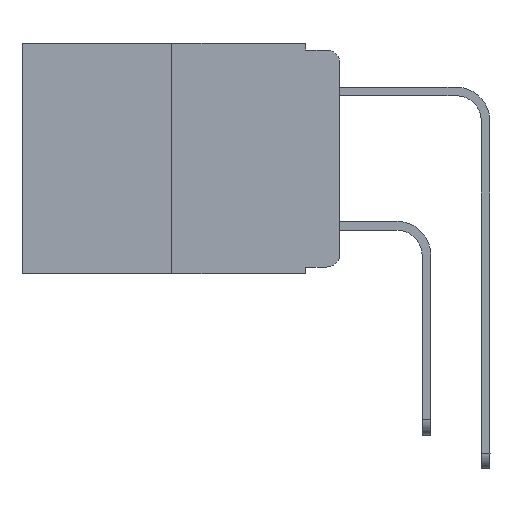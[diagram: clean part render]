
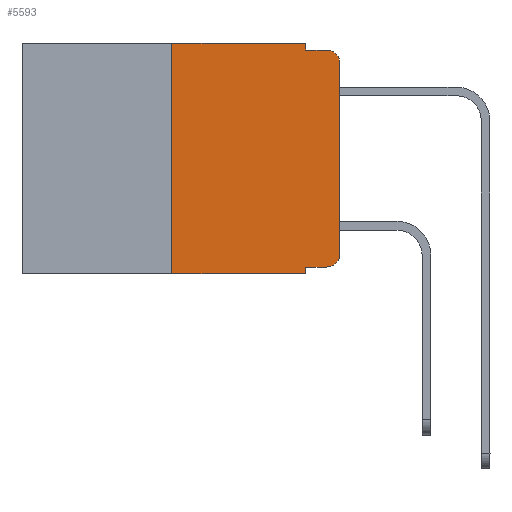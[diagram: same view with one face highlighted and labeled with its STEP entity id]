
A CAD part, left-side view. The second image highlights one B-rep face of the part: STEP entity #5593.
In plain terms, the highlighted planar face has unit normal (-1, 0, 0).
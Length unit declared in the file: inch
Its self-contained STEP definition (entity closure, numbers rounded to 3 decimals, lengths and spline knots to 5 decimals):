
#84 = PLANE ( 'NONE',  #6915 ) ;
#262 = CARTESIAN_POINT ( 'NONE',  ( 0., 0.473, 0. ) ) ;
#278 = DIRECTION ( 'NONE',  ( 0., 0., -1. ) ) ;
#373 = DIRECTION ( 'NONE',  ( 0., 0., 1. ) ) ;
#785 = CARTESIAN_POINT ( 'NONE',  ( 0., 0.473, 0. ) ) ;
#858 = CARTESIAN_POINT ( 'NONE',  ( 0., 0.051, -0.333 ) ) ;
#1084 = CARTESIAN_POINT ( 'NONE',  ( 0., 0., -0.313 ) ) ;
#1629 = LINE ( 'NONE', #12684, #1762 ) ;
#1762 = VECTOR ( 'NONE', #373, 39.37008 ) ;
#1849 = DIRECTION ( 'NONE',  ( 0., 0., -1. ) ) ;
#1924 = VERTEX_POINT ( 'NONE', #5169 ) ;
#2230 = EDGE_CURVE ( 'NONE', #6513, #14766, #7653, .T. ) ;
#2248 = VECTOR ( 'NONE', #9145, 39.37008 ) ;
#2743 = EDGE_CURVE ( 'NONE', #1924, #9829, #5109, .T. ) ;
#2850 = VERTEX_POINT ( 'NONE', #15155 ) ;
#2897 = ORIENTED_EDGE ( 'NONE', *, *, #12793, .T. ) ;
#3230 = CARTESIAN_POINT ( 'NONE',  ( 0., 0., 0. ) ) ;
#3485 = CARTESIAN_POINT ( 'NONE',  ( 0., 0.051, -0.343 ) ) ;
#3687 = ORIENTED_EDGE ( 'NONE', *, *, #15519, .F. ) ;
#3794 = CARTESIAN_POINT ( 'NONE',  ( 0., 0.051, -0.333 ) ) ;
#3809 = ORIENTED_EDGE ( 'NONE', *, *, #9733, .T. ) ;
#4053 = ORIENTED_EDGE ( 'NONE', *, *, #5832, .F. ) ;
#4422 = DIRECTION ( 'NONE',  ( 0., 0., -1. ) ) ;
#4790 = EDGE_CURVE ( 'NONE', #8139, #10326, #15799, .T. ) ;
#4822 = DIRECTION ( 'NONE',  ( 0., 0., -1. ) ) ;
#5012 = EDGE_LOOP ( 'NONE', ( #8319, #14642, #15733, #3687, #16349, #4053, #2897, #10737, #3809, #11576 ) ) ;
#5109 = LINE ( 'NONE', #785, #2248 ) ;
#5169 = CARTESIAN_POINT ( 'NONE',  ( 0., 0.25, 0. ) ) ;
#5593 = ADVANCED_FACE ( 'NONE', ( #11121 ), #84, .F. ) ;
#5717 = DIRECTION ( 'NONE',  ( -1., 0., 0. ) ) ;
#5832 = EDGE_CURVE ( 'NONE', #2850, #1924, #1629, .T. ) ;
#6028 = LINE ( 'NONE', #3230, #13572 ) ;
#6055 = AXIS2_PLACEMENT_3D ( 'NONE', #7145, #5717, #8587 ) ;
#6513 = VERTEX_POINT ( 'NONE', #8680 ) ;
#6915 = AXIS2_PLACEMENT_3D ( 'NONE', #262, #12671, #4422 ) ;
#6958 = VERTEX_POINT ( 'NONE', #12594 ) ;
#7145 = CARTESIAN_POINT ( 'NONE',  ( 0., 0.02, -0.313 ) ) ;
#7242 = CARTESIAN_POINT ( 'NONE',  ( 0., 0.051, 0. ) ) ;
#7386 = LINE ( 'NONE', #17024, #10553 ) ;
#7511 = DIRECTION ( 'NONE',  ( -1., 0., 0. ) ) ;
#7522 = CARTESIAN_POINT ( 'NONE',  ( 0., 0.473, -0.343 ) ) ;
#7631 = EDGE_CURVE ( 'NONE', #10326, #6958, #6028, .T. ) ;
#7653 = LINE ( 'NONE', #14227, #14882 ) ;
#7811 = VECTOR ( 'NONE', #17394, 39.37008 ) ;
#8139 = VERTEX_POINT ( 'NONE', #15971 ) ;
#8319 = ORIENTED_EDGE ( 'NONE', *, *, #7631, .T. ) ;
#8450 = EDGE_CURVE ( 'NONE', #17778, #16083, #11633, .T. ) ;
#8587 = DIRECTION ( 'NONE',  ( 0., 0., -1. ) ) ;
#8680 = CARTESIAN_POINT ( 'NONE',  ( 0., 0.051, -0.01 ) ) ;
#8873 = LINE ( 'NONE', #7522, #12788 ) ;
#8926 = DIRECTION ( 'NONE',  ( 0., -1., 0. ) ) ;
#9145 = DIRECTION ( 'NONE',  ( 0., -1., 0. ) ) ;
#9733 = EDGE_CURVE ( 'NONE', #17778, #8139, #16209, .T. ) ;
#9829 = VERTEX_POINT ( 'NONE', #10786 ) ;
#10132 = VECTOR ( 'NONE', #1849, 39.37008 ) ;
#10326 = VERTEX_POINT ( 'NONE', #1084 ) ;
#10553 = VECTOR ( 'NONE', #278, 39.37008 ) ;
#10737 = ORIENTED_EDGE ( 'NONE', *, *, #8450, .F. ) ;
#10786 = CARTESIAN_POINT ( 'NONE',  ( 0., 0.051, 0. ) ) ;
#11121 = FACE_OUTER_BOUND ( 'NONE', #5012, .T. ) ;
#11576 = ORIENTED_EDGE ( 'NONE', *, *, #4790, .T. ) ;
#11633 = LINE ( 'NONE', #7242, #10132 ) ;
#12594 = CARTESIAN_POINT ( 'NONE',  ( 0., 0., -0.03 ) ) ;
#12671 = DIRECTION ( 'NONE',  ( 1., 0., 0. ) ) ;
#12684 = CARTESIAN_POINT ( 'NONE',  ( 0., 0.25, 0. ) ) ;
#12788 = VECTOR ( 'NONE', #14432, 39.37008 ) ;
#12793 = EDGE_CURVE ( 'NONE', #2850, #16083, #8873, .T. ) ;
#13572 = VECTOR ( 'NONE', #17010, 39.37008 ) ;
#14227 = CARTESIAN_POINT ( 'NONE',  ( 0., 0.051, -0.01 ) ) ;
#14333 = CARTESIAN_POINT ( 'NONE',  ( 0., 0.02, -0.03 ) ) ;
#14432 = DIRECTION ( 'NONE',  ( 0., -1., 0. ) ) ;
#14442 = CARTESIAN_POINT ( 'NONE',  ( 0., 0.02, -0.01 ) ) ;
#14546 = CIRCLE ( 'NONE', #14844, 0.02 ) ;
#14642 = ORIENTED_EDGE ( 'NONE', *, *, #15272, .T. ) ;
#14766 = VERTEX_POINT ( 'NONE', #14442 ) ;
#14844 = AXIS2_PLACEMENT_3D ( 'NONE', #14333, #7511, #4822 ) ;
#14882 = VECTOR ( 'NONE', #8926, 39.37008 ) ;
#15155 = CARTESIAN_POINT ( 'NONE',  ( 0., 0.25, -0.343 ) ) ;
#15272 = EDGE_CURVE ( 'NONE', #6958, #14766, #14546, .T. ) ;
#15519 = EDGE_CURVE ( 'NONE', #9829, #6513, #7386, .T. ) ;
#15733 = ORIENTED_EDGE ( 'NONE', *, *, #2230, .F. ) ;
#15799 = CIRCLE ( 'NONE', #6055, 0.02 ) ;
#15971 = CARTESIAN_POINT ( 'NONE',  ( 0., 0.02, -0.333 ) ) ;
#16083 = VERTEX_POINT ( 'NONE', #3485 ) ;
#16209 = LINE ( 'NONE', #3794, #7811 ) ;
#16349 = ORIENTED_EDGE ( 'NONE', *, *, #2743, .F. ) ;
#17010 = DIRECTION ( 'NONE',  ( 0., 0., 1. ) ) ;
#17024 = CARTESIAN_POINT ( 'NONE',  ( 0., 0.051, 0. ) ) ;
#17394 = DIRECTION ( 'NONE',  ( 0., -1., 0. ) ) ;
#17778 = VERTEX_POINT ( 'NONE', #858 ) ;
